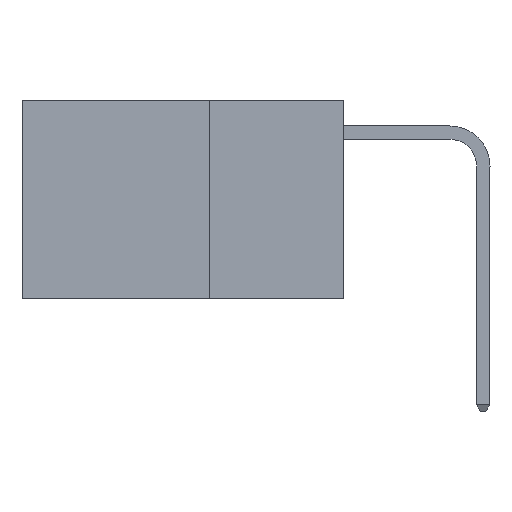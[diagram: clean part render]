
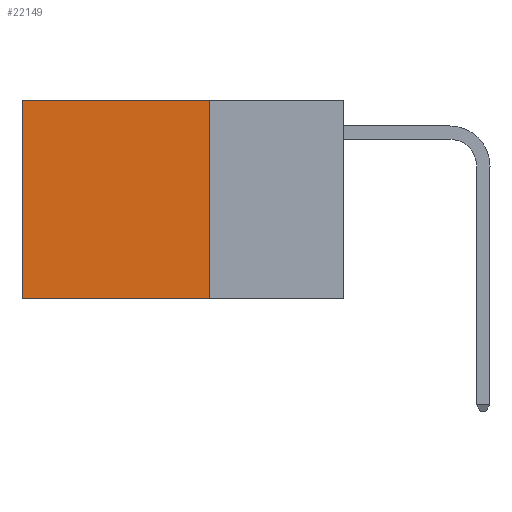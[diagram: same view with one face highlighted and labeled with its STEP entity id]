
A CAD part, left-side view. The second image highlights one B-rep face of the part: STEP entity #22149.
In plain terms, the highlighted planar face has unit normal (-1, 0, 0).
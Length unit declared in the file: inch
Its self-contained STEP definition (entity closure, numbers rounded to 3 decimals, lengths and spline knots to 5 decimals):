
#1324 = CARTESIAN_POINT ( 'NONE',  ( 0.2625, 0.25, 0. ) ) ;
#1363 = DIRECTION ( 'NONE',  ( 0., 1., 0. ) ) ;
#1954 = DIRECTION ( 'NONE',  ( 0., 0., -1. ) ) ;
#2624 = LINE ( 'NONE', #16398, #7499 ) ;
#3415 = DIRECTION ( 'NONE',  ( 1., 0., 0. ) ) ;
#3483 = EDGE_LOOP ( 'NONE', ( #25868, #9915, #9453, #8078 ) ) ;
#3981 = CARTESIAN_POINT ( 'NONE',  ( 0.2625, 0.25, -0.37 ) ) ;
#4265 = EDGE_CURVE ( 'NONE', #12282, #14690, #2624, .T. ) ;
#5260 = EDGE_CURVE ( 'NONE', #23646, #14690, #25353, .T. ) ;
#5317 = CARTESIAN_POINT ( 'NONE',  ( 0.2625, 0.6, 0. ) ) ;
#6179 = CARTESIAN_POINT ( 'NONE',  ( 0.2625, 0.6, -0.37 ) ) ;
#7499 = VECTOR ( 'NONE', #1954, 39.37008 ) ;
#8078 = ORIENTED_EDGE ( 'NONE', *, *, #20380, .T. ) ;
#8359 = VERTEX_POINT ( 'NONE', #14741 ) ;
#9051 = VECTOR ( 'NONE', #21681, 39.37008 ) ;
#9328 = LINE ( 'NONE', #16510, #19608 ) ;
#9453 = ORIENTED_EDGE ( 'NONE', *, *, #16180, .F. ) ;
#9624 = CARTESIAN_POINT ( 'NONE',  ( 0.2625, 0.25, 0. ) ) ;
#9682 = VECTOR ( 'NONE', #1363, 39.37008 ) ;
#9915 = ORIENTED_EDGE ( 'NONE', *, *, #5260, .F. ) ;
#11510 = CARTESIAN_POINT ( 'NONE',  ( 0.2625, 0.25, -0.37 ) ) ;
#12282 = VERTEX_POINT ( 'NONE', #5317 ) ;
#14102 = AXIS2_PLACEMENT_3D ( 'NONE', #1324, #3415, #17830 ) ;
#14421 = FACE_OUTER_BOUND ( 'NONE', #3483, .T. ) ;
#14690 = VERTEX_POINT ( 'NONE', #6179 ) ;
#14741 = CARTESIAN_POINT ( 'NONE',  ( 0.2625, 0.25, 0. ) ) ;
#15782 = PLANE ( 'NONE',  #14102 ) ;
#16180 = EDGE_CURVE ( 'NONE', #8359, #23646, #9328, .T. ) ;
#16398 = CARTESIAN_POINT ( 'NONE',  ( 0.2625, 0.6, 0. ) ) ;
#16510 = CARTESIAN_POINT ( 'NONE',  ( 0.2625, 0.25, 0. ) ) ;
#17830 = DIRECTION ( 'NONE',  ( 0., 0., -1. ) ) ;
#19608 = VECTOR ( 'NONE', #26633, 39.37008 ) ;
#20380 = EDGE_CURVE ( 'NONE', #8359, #12282, #25972, .T. ) ;
#21681 = DIRECTION ( 'NONE',  ( 0., 1., 0. ) ) ;
#22149 = ADVANCED_FACE ( 'NONE', ( #14421 ), #15782, .F. ) ;
#23646 = VERTEX_POINT ( 'NONE', #3981 ) ;
#25353 = LINE ( 'NONE', #11510, #9051 ) ;
#25868 = ORIENTED_EDGE ( 'NONE', *, *, #4265, .T. ) ;
#25972 = LINE ( 'NONE', #9624, #9682 ) ;
#26633 = DIRECTION ( 'NONE',  ( 0., 0., -1. ) ) ;
